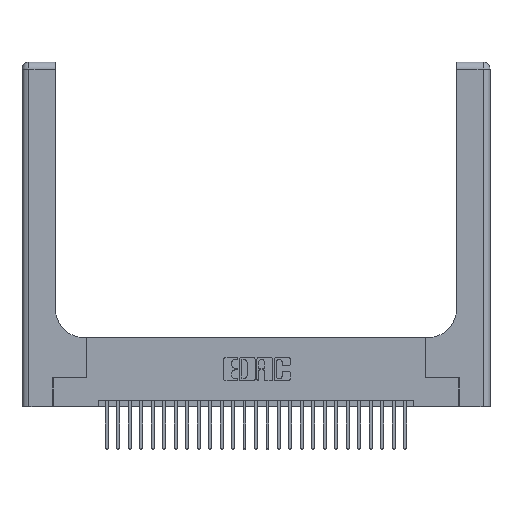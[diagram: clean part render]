
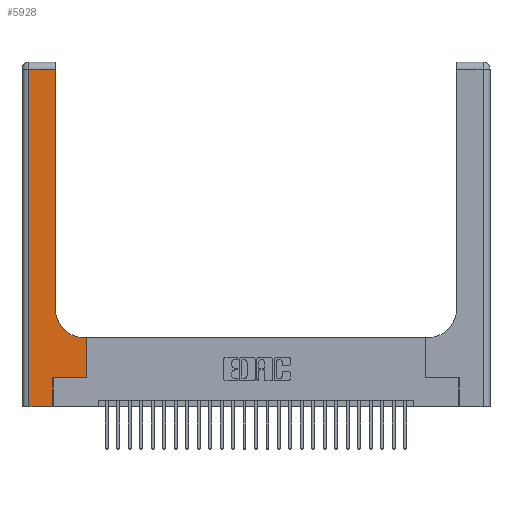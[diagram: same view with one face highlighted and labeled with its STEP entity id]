
A CAD part, top view. The second image highlights one B-rep face of the part: STEP entity #5928.
In plain terms, the highlighted planar face has unit normal (0, 0, 1).
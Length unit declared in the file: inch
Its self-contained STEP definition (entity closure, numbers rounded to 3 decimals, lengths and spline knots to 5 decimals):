
#488 = EDGE_CURVE ( 'NONE', #3143, #14504, #17925, .T. ) ;
#1439 = DIRECTION ( 'NONE',  ( 1., 0., 0. ) ) ;
#1446 = ORIENTED_EDGE ( 'NONE', *, *, #24926, .T. ) ;
#1742 = EDGE_CURVE ( 'NONE', #14504, #8459, #5945, .T. ) ;
#1885 = VECTOR ( 'NONE', #6353, 39.37008 ) ;
#2017 = VECTOR ( 'NONE', #17922, 39.37008 ) ;
#2804 = ORIENTED_EDGE ( 'NONE', *, *, #23829, .T. ) ;
#3010 = CARTESIAN_POINT ( 'NONE',  ( 0.06, 3., 0.37 ) ) ;
#3143 = VERTEX_POINT ( 'NONE', #27565 ) ;
#3829 = VERTEX_POINT ( 'NONE', #7197 ) ;
#3863 = PLANE ( 'NONE',  #8364 ) ;
#3945 = LINE ( 'NONE', #18191, #25887 ) ;
#3985 = CARTESIAN_POINT ( 'NONE',  ( 0., 0., 0.37 ) ) ;
#4670 = LINE ( 'NONE', #22290, #27633 ) ;
#4727 = CARTESIAN_POINT ( 'NONE',  ( 0.2915, 2.94, 0.37 ) ) ;
#4876 = DIRECTION ( 'NONE',  ( 0., 1., 0. ) ) ;
#5255 = ORIENTED_EDGE ( 'NONE', *, *, #22145, .T. ) ;
#5928 = ADVANCED_FACE ( 'NONE', ( #17980 ), #3863, .F. ) ;
#5945 = LINE ( 'NONE', #17990, #12480 ) ;
#6353 = DIRECTION ( 'NONE',  ( 1., 0., 0. ) ) ;
#6455 = DIRECTION ( 'NONE',  ( 0., 0., -1. ) ) ;
#6789 = CARTESIAN_POINT ( 'NONE',  ( 0.269, 0., 0.37 ) ) ;
#7154 = LINE ( 'NONE', #3010, #2017 ) ;
#7197 = CARTESIAN_POINT ( 'NONE',  ( 0.06, 2.94, 0.37 ) ) ;
#7203 = CARTESIAN_POINT ( 'NONE',  ( 0.5585, 0.6, 0.37 ) ) ;
#7643 = VECTOR ( 'NONE', #1439, 39.37008 ) ;
#7648 = CARTESIAN_POINT ( 'NONE',  ( 0.06, 0., 0.37 ) ) ;
#7715 = LINE ( 'NONE', #3985, #1885 ) ;
#8063 = DIRECTION ( 'NONE',  ( -1., 0., 0. ) ) ;
#8364 = AXIS2_PLACEMENT_3D ( 'NONE', #28025, #25415, #21010 ) ;
#8459 = VERTEX_POINT ( 'NONE', #4727 ) ;
#8808 = ORIENTED_EDGE ( 'NONE', *, *, #15554, .T. ) ;
#8984 = DIRECTION ( 'NONE',  ( -1., 0., 0. ) ) ;
#9884 = EDGE_CURVE ( 'NONE', #13211, #21656, #25146, .T. ) ;
#10009 = LINE ( 'NONE', #18853, #21735 ) ;
#10012 = CARTESIAN_POINT ( 'NONE',  ( 0.5585, 0.25, 0.37 ) ) ;
#10562 = VERTEX_POINT ( 'NONE', #6789 ) ;
#10858 = DIRECTION ( 'NONE',  ( 1., 0., 0. ) ) ;
#11200 = CARTESIAN_POINT ( 'NONE',  ( 0.2915, 0.6, 0.37 ) ) ;
#11332 = EDGE_LOOP ( 'NONE', ( #24637, #19766, #5255, #1446, #26981, #14137, #8808, #2804, #15294 ) ) ;
#12480 = VECTOR ( 'NONE', #22417, 39.37008 ) ;
#12925 = LINE ( 'NONE', #11200, #14275 ) ;
#13211 = VERTEX_POINT ( 'NONE', #19155 ) ;
#14137 = ORIENTED_EDGE ( 'NONE', *, *, #9884, .T. ) ;
#14275 = VECTOR ( 'NONE', #8984, 39.37008 ) ;
#14504 = VERTEX_POINT ( 'NONE', #14654 ) ;
#14654 = CARTESIAN_POINT ( 'NONE',  ( 0.2915, 0.85, 0.37 ) ) ;
#15294 = ORIENTED_EDGE ( 'NONE', *, *, #488, .T. ) ;
#15554 = EDGE_CURVE ( 'NONE', #21656, #17073, #4670, .T. ) ;
#16177 = DIRECTION ( 'NONE',  ( 0., 1., 0. ) ) ;
#17073 = VERTEX_POINT ( 'NONE', #7203 ) ;
#17590 = EDGE_CURVE ( 'NONE', #8459, #3829, #10009, .T. ) ;
#17783 = VERTEX_POINT ( 'NONE', #7648 ) ;
#17922 = DIRECTION ( 'NONE',  ( 0., -1., 0. ) ) ;
#17925 = CIRCLE ( 'NONE', #18689, 0.25 ) ;
#17980 = FACE_OUTER_BOUND ( 'NONE', #11332, .T. ) ;
#17990 = CARTESIAN_POINT ( 'NONE',  ( 0.2915, 3., 0.37 ) ) ;
#18191 = CARTESIAN_POINT ( 'NONE',  ( 0.269, 0., 0.37 ) ) ;
#18689 = AXIS2_PLACEMENT_3D ( 'NONE', #19571, #6455, #10858 ) ;
#18853 = CARTESIAN_POINT ( 'NONE',  ( 0., 2.94, 0.37 ) ) ;
#19155 = CARTESIAN_POINT ( 'NONE',  ( 0.269, 0.25, 0.37 ) ) ;
#19571 = CARTESIAN_POINT ( 'NONE',  ( 0.5415, 0.85, 0.37 ) ) ;
#19766 = ORIENTED_EDGE ( 'NONE', *, *, #17590, .T. ) ;
#21010 = DIRECTION ( 'NONE',  ( -1., 0., 0. ) ) ;
#21656 = VERTEX_POINT ( 'NONE', #10012 ) ;
#21735 = VECTOR ( 'NONE', #8063, 39.37008 ) ;
#22145 = EDGE_CURVE ( 'NONE', #3829, #17783, #7154, .T. ) ;
#22290 = CARTESIAN_POINT ( 'NONE',  ( 0.5585, 0.25, 0.37 ) ) ;
#22417 = DIRECTION ( 'NONE',  ( 0., 1., 0. ) ) ;
#23829 = EDGE_CURVE ( 'NONE', #17073, #3143, #12925, .T. ) ;
#24637 = ORIENTED_EDGE ( 'NONE', *, *, #1742, .T. ) ;
#24926 = EDGE_CURVE ( 'NONE', #17783, #10562, #7715, .T. ) ;
#25100 = EDGE_CURVE ( 'NONE', #10562, #13211, #3945, .T. ) ;
#25146 = LINE ( 'NONE', #27821, #7643 ) ;
#25415 = DIRECTION ( 'NONE',  ( 0., 0., -1. ) ) ;
#25887 = VECTOR ( 'NONE', #16177, 39.37008 ) ;
#26981 = ORIENTED_EDGE ( 'NONE', *, *, #25100, .T. ) ;
#27565 = CARTESIAN_POINT ( 'NONE',  ( 0.5415, 0.6, 0.37 ) ) ;
#27633 = VECTOR ( 'NONE', #4876, 39.37008 ) ;
#27821 = CARTESIAN_POINT ( 'NONE',  ( 0.269, 0.25, 0.37 ) ) ;
#28025 = CARTESIAN_POINT ( 'NONE',  ( 0., 3., 0.37 ) ) ;
